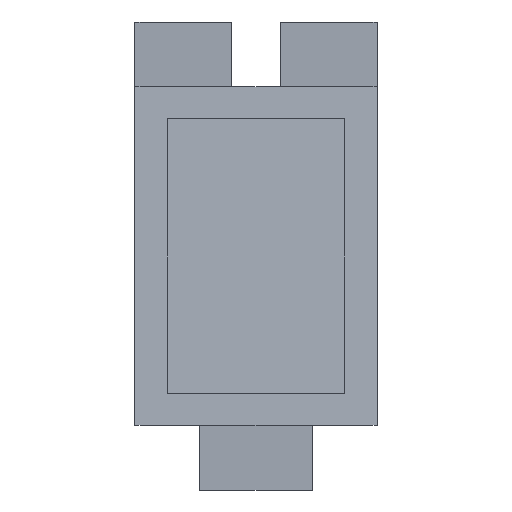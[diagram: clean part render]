
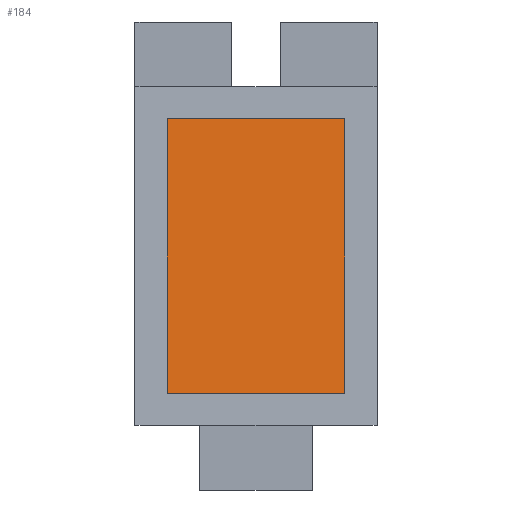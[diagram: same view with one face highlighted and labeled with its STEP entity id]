
A CAD part, front view. The second image highlights one B-rep face of the part: STEP entity #184.
In plain terms, the highlighted planar face has unit normal (0, -0.996, 0.095).
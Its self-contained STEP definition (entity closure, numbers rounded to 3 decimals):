
#3 = VERTEX_POINT ( 'NONE', #908 ) ;
#26 = ORIENTED_EDGE ( 'NONE', *, *, #28, .T. ) ;
#28 = EDGE_CURVE ( 'NONE', #496, #289, #907, .T. ) ;
#50 = ORIENTED_EDGE ( 'NONE', *, *, #533, .T. ) ;
#58 = ORIENTED_EDGE ( 'NONE', *, *, #663, .T. ) ;
#91 = EDGE_CURVE ( 'NONE', #95, #3, #865, .T. ) ;
#95 = VERTEX_POINT ( 'NONE', #635 ) ;
#184 = ADVANCED_FACE ( 'NONE', ( #762 ), #361, .F. ) ;
#218 = CARTESIAN_POINT ( 'NONE',  ( 58.125, 125.409, -162.332 ) ) ;
#225 = ORIENTED_EDGE ( 'NONE', *, *, #91, .T. ) ;
#289 = VERTEX_POINT ( 'NONE', #838 ) ;
#307 = DIRECTION ( 'NONE',  ( 0., 0.995, -0.095 ) ) ;
#334 = EDGE_LOOP ( 'NONE', ( #225, #58, #26, #50 ) ) ;
#359 = DIRECTION ( 'NONE',  ( 0., 0.095, 0.995 ) ) ;
#361 = PLANE ( 'NONE',  #450 ) ;
#367 = CARTESIAN_POINT ( 'NONE',  ( 9.375, 136.966, -40.981 ) ) ;
#385 = CARTESIAN_POINT ( 'NONE',  ( 16.875, 125.409, -162.332 ) ) ;
#403 = DIRECTION ( 'NONE',  ( 1., 0., 0. ) ) ;
#408 = VECTOR ( 'NONE', #403, 1000. ) ;
#410 = LINE ( 'NONE', #385, #408 ) ;
#450 = AXIS2_PLACEMENT_3D ( 'NONE', #367, #307, #359 ) ;
#465 = VECTOR ( 'NONE', #491, 1000. ) ;
#482 = LINE ( 'NONE', #501, #465 ) ;
#491 = DIRECTION ( 'NONE',  ( -1., 0., 0. ) ) ;
#496 = VERTEX_POINT ( 'NONE', #218 ) ;
#501 = CARTESIAN_POINT ( 'NONE',  ( 16.875, 131.487, -98.514 ) ) ;
#533 = EDGE_CURVE ( 'NONE', #289, #95, #482, .T. ) ;
#603 = CARTESIAN_POINT ( 'NONE',  ( 16.875, 125.409, -162.332 ) ) ;
#635 = CARTESIAN_POINT ( 'NONE',  ( 16.875, 131.487, -98.514 ) ) ;
#653 = DIRECTION ( 'NONE',  ( 0., -0.095, -0.995 ) ) ;
#663 = EDGE_CURVE ( 'NONE', #3, #496, #410, .T. ) ;
#762 = FACE_OUTER_BOUND ( 'NONE', #334, .T. ) ;
#809 = DIRECTION ( 'NONE',  ( 0., 0.095, 0.995 ) ) ;
#826 = VECTOR ( 'NONE', #653, 1000. ) ;
#838 = CARTESIAN_POINT ( 'NONE',  ( 58.125, 131.487, -98.514 ) ) ;
#865 = LINE ( 'NONE', #603, #826 ) ;
#880 = VECTOR ( 'NONE', #809, 1000. ) ;
#907 = LINE ( 'NONE', #910, #880 ) ;
#908 = CARTESIAN_POINT ( 'NONE',  ( 16.875, 125.409, -162.332 ) ) ;
#910 = CARTESIAN_POINT ( 'NONE',  ( 58.125, 125.409, -162.332 ) ) ;
